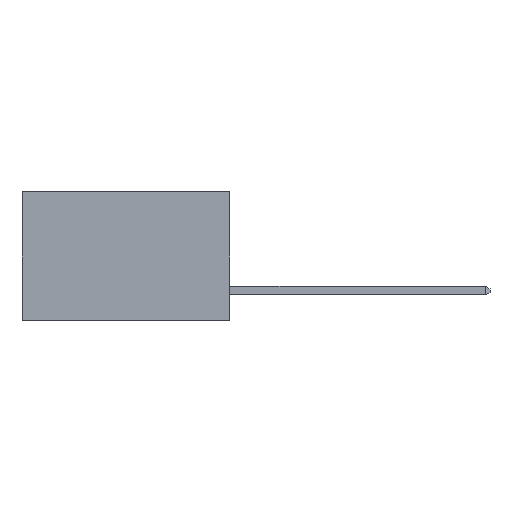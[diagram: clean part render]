
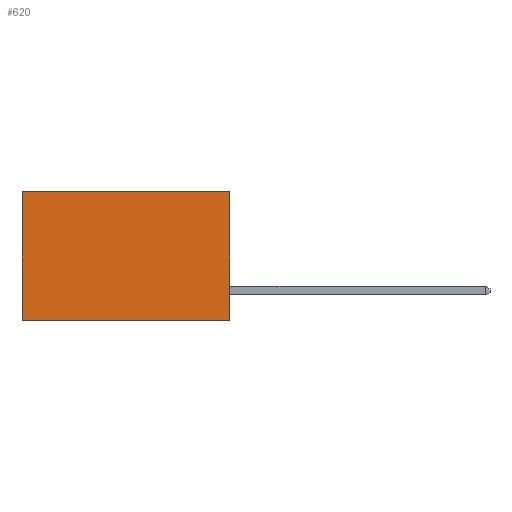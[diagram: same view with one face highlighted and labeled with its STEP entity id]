
A CAD part, left-side view. The second image highlights one B-rep face of the part: STEP entity #620.
In plain terms, the highlighted planar face has unit normal (-1, 0, 0).
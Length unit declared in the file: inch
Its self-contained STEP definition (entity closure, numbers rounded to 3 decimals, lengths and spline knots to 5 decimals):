
#620 = ADVANCED_FACE ( 'NONE', ( #1708 ), #2516, .F. ) ;
#1055 = VERTEX_POINT ( 'NONE', #7873 ) ;
#1609 = CARTESIAN_POINT ( 'NONE',  ( 0.2615, 0., 0. ) ) ;
#1674 = DIRECTION ( 'NONE',  ( 0., 0., -1. ) ) ;
#1708 = FACE_OUTER_BOUND ( 'NONE', #10484, .T. ) ;
#1723 = CARTESIAN_POINT ( 'NONE',  ( 0.2615, 0., -0.37 ) ) ;
#1990 = DIRECTION ( 'NONE',  ( 1., 0., 0. ) ) ;
#2516 = PLANE ( 'NONE',  #8050 ) ;
#3397 = ORIENTED_EDGE ( 'NONE', *, *, #10439, .T. ) ;
#3450 = EDGE_CURVE ( 'NONE', #1055, #11088, #5198, .T. ) ;
#3873 = DIRECTION ( 'NONE',  ( 0., 1., 0. ) ) ;
#4027 = CARTESIAN_POINT ( 'NONE',  ( 0.2615, 0., -0.37 ) ) ;
#4735 = VECTOR ( 'NONE', #10911, 39.37008 ) ;
#4970 = CARTESIAN_POINT ( 'NONE',  ( 0.2615, 0., -0.37 ) ) ;
#5118 = ORIENTED_EDGE ( 'NONE', *, *, #8976, .F. ) ;
#5198 = LINE ( 'NONE', #6217, #7290 ) ;
#5274 = VERTEX_POINT ( 'NONE', #1609 ) ;
#5389 = VERTEX_POINT ( 'NONE', #4970 ) ;
#6217 = CARTESIAN_POINT ( 'NONE',  ( 0.2615, 0.6, -0.37 ) ) ;
#7012 = DIRECTION ( 'NONE',  ( 0., 0., -1. ) ) ;
#7034 = ORIENTED_EDGE ( 'NONE', *, *, #3450, .T. ) ;
#7290 = VECTOR ( 'NONE', #1674, 39.37008 ) ;
#7304 = LINE ( 'NONE', #1723, #11495 ) ;
#7418 = LINE ( 'NONE', #10064, #11869 ) ;
#7873 = CARTESIAN_POINT ( 'NONE',  ( 0.2615, 0.6, 0. ) ) ;
#8050 = AXIS2_PLACEMENT_3D ( 'NONE', #4027, #1990, #7012 ) ;
#8976 = EDGE_CURVE ( 'NONE', #5389, #11088, #7304, .T. ) ;
#9071 = CARTESIAN_POINT ( 'NONE',  ( 0.2615, 0.6, -0.37 ) ) ;
#9342 = DIRECTION ( 'NONE',  ( 0., 1., 0. ) ) ;
#10064 = CARTESIAN_POINT ( 'NONE',  ( 0.2615, 0., 0. ) ) ;
#10439 = EDGE_CURVE ( 'NONE', #5274, #1055, #7418, .T. ) ;
#10464 = EDGE_CURVE ( 'NONE', #5274, #5389, #11600, .T. ) ;
#10484 = EDGE_LOOP ( 'NONE', ( #7034, #5118, #11952, #3397 ) ) ;
#10911 = DIRECTION ( 'NONE',  ( 0., 0., -1. ) ) ;
#11088 = VERTEX_POINT ( 'NONE', #9071 ) ;
#11495 = VECTOR ( 'NONE', #9342, 39.37008 ) ;
#11600 = LINE ( 'NONE', #11708, #4735 ) ;
#11708 = CARTESIAN_POINT ( 'NONE',  ( 0.2615, 0., -0.37 ) ) ;
#11869 = VECTOR ( 'NONE', #3873, 39.37008 ) ;
#11952 = ORIENTED_EDGE ( 'NONE', *, *, #10464, .F. ) ;
